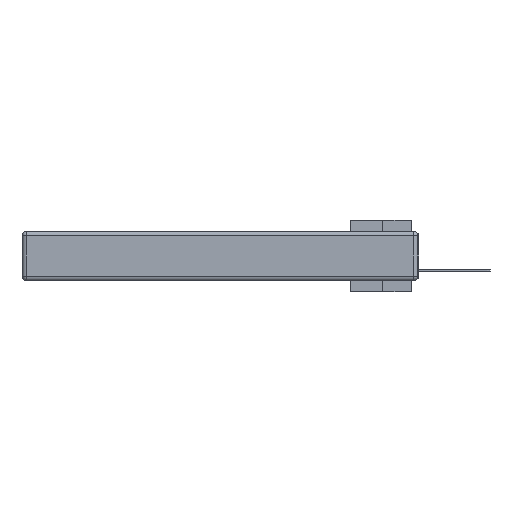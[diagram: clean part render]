
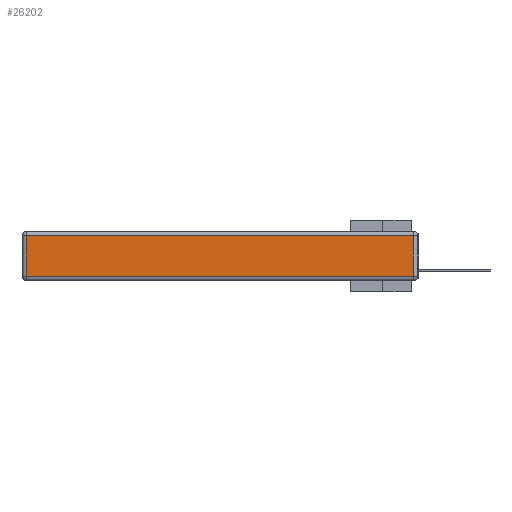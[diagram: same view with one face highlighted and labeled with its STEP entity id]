
A CAD part, left-side view. The second image highlights one B-rep face of the part: STEP entity #26202.
In plain terms, the highlighted planar face has unit normal (-1, 0, 0).
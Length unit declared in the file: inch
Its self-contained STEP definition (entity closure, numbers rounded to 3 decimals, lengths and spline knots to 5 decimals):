
#563 = ORIENTED_EDGE ( 'NONE', *, *, #8029, .T. ) ;
#1807 = VERTEX_POINT ( 'NONE', #12797 ) ;
#1899 = CARTESIAN_POINT ( 'NONE',  ( 0., 0.03, -0.343 ) ) ;
#3553 = CARTESIAN_POINT ( 'NONE',  ( 0., 2.75, -0.03 ) ) ;
#4404 = VECTOR ( 'NONE', #27000, 39.37008 ) ;
#4785 = EDGE_LOOP ( 'NONE', ( #14831, #563, #30669, #7475 ) ) ;
#4827 = FACE_OUTER_BOUND ( 'NONE', #4785, .T. ) ;
#6003 = CARTESIAN_POINT ( 'NONE',  ( 0., 2.72, -0.03 ) ) ;
#7202 = CARTESIAN_POINT ( 'NONE',  ( 0., 2.72, -0.343 ) ) ;
#7475 = ORIENTED_EDGE ( 'NONE', *, *, #24902, .T. ) ;
#8029 = EDGE_CURVE ( 'NONE', #1807, #29906, #9313, .T. ) ;
#8271 = VECTOR ( 'NONE', #28703, 39.37008 ) ;
#8482 = DIRECTION ( 'NONE',  ( -1., 0., 0. ) ) ;
#9313 = LINE ( 'NONE', #1899, #26384 ) ;
#9468 = DIRECTION ( 'NONE',  ( 0., 0., 1. ) ) ;
#10370 = AXIS2_PLACEMENT_3D ( 'NONE', #28774, #8482, #23771 ) ;
#12173 = VECTOR ( 'NONE', #31478, 39.37008 ) ;
#12797 = CARTESIAN_POINT ( 'NONE',  ( 0., 0.03, -0.313 ) ) ;
#12920 = LINE ( 'NONE', #7202, #12173 ) ;
#13692 = EDGE_CURVE ( 'NONE', #29906, #29705, #17200, .T. ) ;
#14831 = ORIENTED_EDGE ( 'NONE', *, *, #21649, .T. ) ;
#17200 = LINE ( 'NONE', #3553, #8271 ) ;
#21649 = EDGE_CURVE ( 'NONE', #22437, #1807, #23380, .T. ) ;
#22437 = VERTEX_POINT ( 'NONE', #24598 ) ;
#23380 = LINE ( 'NONE', #29383, #4404 ) ;
#23771 = DIRECTION ( 'NONE',  ( 0., 0., 1. ) ) ;
#24598 = CARTESIAN_POINT ( 'NONE',  ( 0., 2.72, -0.313 ) ) ;
#24902 = EDGE_CURVE ( 'NONE', #29705, #22437, #12920, .T. ) ;
#26202 = ADVANCED_FACE ( 'NONE', ( #4827 ), #30703, .T. ) ;
#26384 = VECTOR ( 'NONE', #9468, 39.37008 ) ;
#26843 = CARTESIAN_POINT ( 'NONE',  ( 0., 0.03, -0.03 ) ) ;
#27000 = DIRECTION ( 'NONE',  ( 0., -1., 0. ) ) ;
#28703 = DIRECTION ( 'NONE',  ( 0., 1., 0. ) ) ;
#28774 = CARTESIAN_POINT ( 'NONE',  ( 0., 0., -0.343 ) ) ;
#29383 = CARTESIAN_POINT ( 'NONE',  ( 0., 0., -0.313 ) ) ;
#29705 = VERTEX_POINT ( 'NONE', #6003 ) ;
#29906 = VERTEX_POINT ( 'NONE', #26843 ) ;
#30669 = ORIENTED_EDGE ( 'NONE', *, *, #13692, .T. ) ;
#30703 = PLANE ( 'NONE',  #10370 ) ;
#31478 = DIRECTION ( 'NONE',  ( 0., 0., -1. ) ) ;
